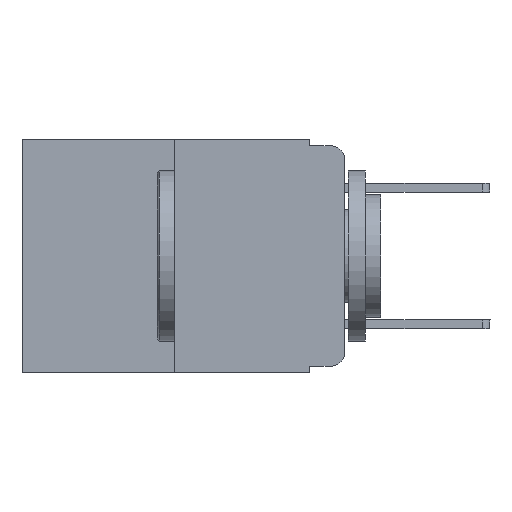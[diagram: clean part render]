
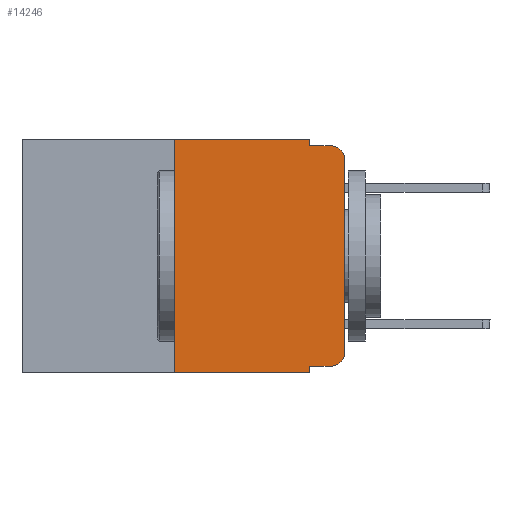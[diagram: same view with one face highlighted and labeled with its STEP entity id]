
A CAD part, left-side view. The second image highlights one B-rep face of the part: STEP entity #14246.
In plain terms, the highlighted planar face has unit normal (-1, 0, 0).
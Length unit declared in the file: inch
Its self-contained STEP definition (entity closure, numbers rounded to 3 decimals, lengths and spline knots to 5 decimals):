
#916 = DIRECTION ( 'NONE',  ( 0., -1., 0. ) ) ;
#934 = VERTEX_POINT ( 'NONE', #12264 ) ;
#1136 = CARTESIAN_POINT ( 'NONE',  ( 0., 0.051, 0. ) ) ;
#1240 = EDGE_CURVE ( 'NONE', #3278, #934, #13041, .T. ) ;
#1336 = VERTEX_POINT ( 'NONE', #14059 ) ;
#2493 = CARTESIAN_POINT ( 'NONE',  ( 0., 0.02, -0.03 ) ) ;
#2527 = LINE ( 'NONE', #12313, #9939 ) ;
#3095 = VERTEX_POINT ( 'NONE', #3627 ) ;
#3278 = VERTEX_POINT ( 'NONE', #9200 ) ;
#3329 = CARTESIAN_POINT ( 'NONE',  ( 0., 0.473, 0. ) ) ;
#3627 = CARTESIAN_POINT ( 'NONE',  ( 0., 0.051, -0.343 ) ) ;
#3693 = DIRECTION ( 'NONE',  ( -1., 0., 0. ) ) ;
#3744 = DIRECTION ( 'NONE',  ( -1., 0., 0. ) ) ;
#3903 = DIRECTION ( 'NONE',  ( 0., 0., 1. ) ) ;
#4099 = DIRECTION ( 'NONE',  ( 0., 0., -1. ) ) ;
#4244 = CARTESIAN_POINT ( 'NONE',  ( 0., 0., 0. ) ) ;
#4460 = CARTESIAN_POINT ( 'NONE',  ( 0., 0.051, -0.333 ) ) ;
#4653 = DIRECTION ( 'NONE',  ( 1., 0., 0. ) ) ;
#4750 = CARTESIAN_POINT ( 'NONE',  ( 0., 0.02, -0.01 ) ) ;
#4943 = AXIS2_PLACEMENT_3D ( 'NONE', #3329, #4653, #6229 ) ;
#5284 = CARTESIAN_POINT ( 'NONE',  ( 0., 0.051, 0. ) ) ;
#5348 = VECTOR ( 'NONE', #4099, 39.37008 ) ;
#5415 = VECTOR ( 'NONE', #916, 39.37008 ) ;
#5568 = ORIENTED_EDGE ( 'NONE', *, *, #16421, .F. ) ;
#5686 = VECTOR ( 'NONE', #14892, 39.37008 ) ;
#6229 = DIRECTION ( 'NONE',  ( 0., 0., -1. ) ) ;
#7476 = VERTEX_POINT ( 'NONE', #11110 ) ;
#7676 = LINE ( 'NONE', #13494, #8324 ) ;
#7862 = ORIENTED_EDGE ( 'NONE', *, *, #14862, .T. ) ;
#8133 = EDGE_CURVE ( 'NONE', #8821, #3095, #13935, .T. ) ;
#8143 = CARTESIAN_POINT ( 'NONE',  ( 0., 0.051, -0.01 ) ) ;
#8324 = VECTOR ( 'NONE', #3903, 39.37008 ) ;
#8603 = ORIENTED_EDGE ( 'NONE', *, *, #12795, .T. ) ;
#8662 = DIRECTION ( 'NONE',  ( 0., 0., 1. ) ) ;
#8729 = LINE ( 'NONE', #4460, #13889 ) ;
#8753 = ORIENTED_EDGE ( 'NONE', *, *, #12741, .T. ) ;
#8774 = DIRECTION ( 'NONE',  ( 0., -1., 0. ) ) ;
#8821 = VERTEX_POINT ( 'NONE', #10094 ) ;
#8936 = LINE ( 'NONE', #5284, #5348 ) ;
#9200 = CARTESIAN_POINT ( 'NONE',  ( 0., 0., -0.313 ) ) ;
#9240 = VERTEX_POINT ( 'NONE', #11454 ) ;
#9622 = EDGE_LOOP ( 'NONE', ( #10313, #7862, #16809, #14337, #11290, #5568, #8603, #11359, #9882, #8753 ) ) ;
#9696 = AXIS2_PLACEMENT_3D ( 'NONE', #10567, #3744, #13259 ) ;
#9882 = ORIENTED_EDGE ( 'NONE', *, *, #17410, .T. ) ;
#9884 = FACE_OUTER_BOUND ( 'NONE', #9622, .T. ) ;
#9939 = VECTOR ( 'NONE', #10983, 39.37008 ) ;
#10094 = CARTESIAN_POINT ( 'NONE',  ( 0., 0.051, -0.333 ) ) ;
#10165 = VERTEX_POINT ( 'NONE', #1136 ) ;
#10313 = ORIENTED_EDGE ( 'NONE', *, *, #1240, .T. ) ;
#10464 = EDGE_CURVE ( 'NONE', #10165, #14457, #8936, .T. ) ;
#10567 = CARTESIAN_POINT ( 'NONE',  ( 0., 0.02, -0.313 ) ) ;
#10696 = CARTESIAN_POINT ( 'NONE',  ( 0., 0.473, -0.343 ) ) ;
#10983 = DIRECTION ( 'NONE',  ( 0., -1., 0. ) ) ;
#11094 = VECTOR ( 'NONE', #8662, 39.37008 ) ;
#11110 = CARTESIAN_POINT ( 'NONE',  ( 0., 0.02, -0.333 ) ) ;
#11290 = ORIENTED_EDGE ( 'NONE', *, *, #14005, .F. ) ;
#11359 = ORIENTED_EDGE ( 'NONE', *, *, #8133, .F. ) ;
#11454 = CARTESIAN_POINT ( 'NONE',  ( 0., 0.25, -0.343 ) ) ;
#11550 = PLANE ( 'NONE',  #4943 ) ;
#12192 = DIRECTION ( 'NONE',  ( 0., 0., -1. ) ) ;
#12264 = CARTESIAN_POINT ( 'NONE',  ( 0., 0., -0.03 ) ) ;
#12311 = LINE ( 'NONE', #10696, #5686 ) ;
#12313 = CARTESIAN_POINT ( 'NONE',  ( 0., 0.473, 0. ) ) ;
#12741 = EDGE_CURVE ( 'NONE', #7476, #3278, #15318, .T. ) ;
#12795 = EDGE_CURVE ( 'NONE', #9240, #3095, #12311, .T. ) ;
#13041 = LINE ( 'NONE', #4244, #11094 ) ;
#13259 = DIRECTION ( 'NONE',  ( 0., 0., -1. ) ) ;
#13402 = CARTESIAN_POINT ( 'NONE',  ( 0., 0.051, -0.01 ) ) ;
#13494 = CARTESIAN_POINT ( 'NONE',  ( 0., 0.25, 0. ) ) ;
#13740 = AXIS2_PLACEMENT_3D ( 'NONE', #2493, #3693, #15924 ) ;
#13889 = VECTOR ( 'NONE', #8774, 39.37008 ) ;
#13935 = LINE ( 'NONE', #17678, #15673 ) ;
#14005 = EDGE_CURVE ( 'NONE', #1336, #10165, #2527, .T. ) ;
#14059 = CARTESIAN_POINT ( 'NONE',  ( 0., 0.25, 0. ) ) ;
#14246 = ADVANCED_FACE ( 'NONE', ( #9884 ), #11550, .F. ) ;
#14337 = ORIENTED_EDGE ( 'NONE', *, *, #10464, .F. ) ;
#14381 = LINE ( 'NONE', #13402, #5415 ) ;
#14457 = VERTEX_POINT ( 'NONE', #8143 ) ;
#14862 = EDGE_CURVE ( 'NONE', #934, #17528, #16707, .T. ) ;
#14892 = DIRECTION ( 'NONE',  ( 0., -1., 0. ) ) ;
#14956 = EDGE_CURVE ( 'NONE', #14457, #17528, #14381, .T. ) ;
#15318 = CIRCLE ( 'NONE', #9696, 0.02 ) ;
#15673 = VECTOR ( 'NONE', #12192, 39.37008 ) ;
#15924 = DIRECTION ( 'NONE',  ( 0., 0., -1. ) ) ;
#16421 = EDGE_CURVE ( 'NONE', #9240, #1336, #7676, .T. ) ;
#16707 = CIRCLE ( 'NONE', #13740, 0.02 ) ;
#16809 = ORIENTED_EDGE ( 'NONE', *, *, #14956, .F. ) ;
#17410 = EDGE_CURVE ( 'NONE', #8821, #7476, #8729, .T. ) ;
#17528 = VERTEX_POINT ( 'NONE', #4750 ) ;
#17678 = CARTESIAN_POINT ( 'NONE',  ( 0., 0.051, 0. ) ) ;
